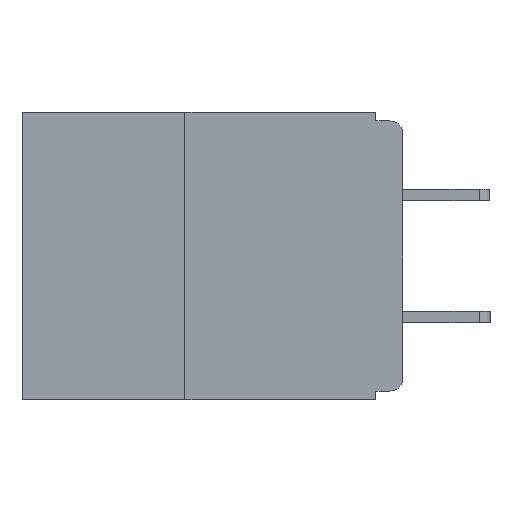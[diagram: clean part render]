
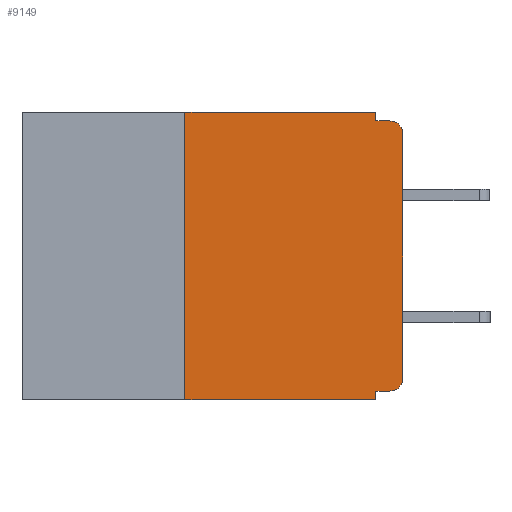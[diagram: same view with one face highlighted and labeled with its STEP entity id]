
A CAD part, left-side view. The second image highlights one B-rep face of the part: STEP entity #9149.
In plain terms, the highlighted planar face has unit normal (-1, 0, 0).
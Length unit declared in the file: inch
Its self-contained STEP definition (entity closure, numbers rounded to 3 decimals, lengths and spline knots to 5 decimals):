
#186 = CARTESIAN_POINT ( 'NONE',  ( 0., 0.25, -0.33 ) ) ;
#391 = DIRECTION ( 'NONE',  ( 0., -1., 0. ) ) ;
#554 = VECTOR ( 'NONE', #391, 39.37008 ) ;
#640 = DIRECTION ( 'NONE',  ( 0., 0., -1. ) ) ;
#1594 = ORIENTED_EDGE ( 'NONE', *, *, #13104, .F. ) ;
#1728 = DIRECTION ( 'NONE',  ( -1., 0., 0. ) ) ;
#1884 = DIRECTION ( 'NONE',  ( 0., 0., -1. ) ) ;
#1994 = CARTESIAN_POINT ( 'NONE',  ( 0., 0.031, -0.33 ) ) ;
#2192 = EDGE_CURVE ( 'NONE', #4188, #13887, #20317, .T. ) ;
#3362 = FACE_OUTER_BOUND ( 'NONE', #13336, .T. ) ;
#3579 = CARTESIAN_POINT ( 'NONE',  ( 0., 0., 0. ) ) ;
#3636 = VERTEX_POINT ( 'NONE', #9568 ) ;
#4188 = VERTEX_POINT ( 'NONE', #186 ) ;
#4613 = CARTESIAN_POINT ( 'NONE',  ( 0., 0.031, -0.01 ) ) ;
#4801 = CARTESIAN_POINT ( 'NONE',  ( 0., 0.015, -0.01 ) ) ;
#4860 = VECTOR ( 'NONE', #6472, 39.37008 ) ;
#4963 = EDGE_CURVE ( 'NONE', #12158, #17159, #18453, .T. ) ;
#5344 = EDGE_CURVE ( 'NONE', #3636, #17159, #9662, .T. ) ;
#6129 = VERTEX_POINT ( 'NONE', #19874 ) ;
#6215 = ORIENTED_EDGE ( 'NONE', *, *, #6844, .T. ) ;
#6323 = VECTOR ( 'NONE', #7617, 39.37008 ) ;
#6472 = DIRECTION ( 'NONE',  ( 0., 1., 0. ) ) ;
#6796 = ORIENTED_EDGE ( 'NONE', *, *, #16630, .F. ) ;
#6844 = EDGE_CURVE ( 'NONE', #16861, #6129, #16753, .T. ) ;
#7011 = VECTOR ( 'NONE', #11040, 39.37008 ) ;
#7360 = CARTESIAN_POINT ( 'NONE',  ( 0., 0.437, 0. ) ) ;
#7577 = LINE ( 'NONE', #1994, #7011 ) ;
#7617 = DIRECTION ( 'NONE',  ( 0., -1., 0. ) ) ;
#7677 = DIRECTION ( 'NONE',  ( -1., 0., 0. ) ) ;
#7740 = VECTOR ( 'NONE', #640, 39.37008 ) ;
#7814 = VECTOR ( 'NONE', #16091, 39.37008 ) ;
#8585 = VECTOR ( 'NONE', #15892, 39.37008 ) ;
#8805 = ORIENTED_EDGE ( 'NONE', *, *, #2192, .T. ) ;
#8962 = VERTEX_POINT ( 'NONE', #12191 ) ;
#9127 = LINE ( 'NONE', #22198, #4860 ) ;
#9149 = ADVANCED_FACE ( 'NONE', ( #3362 ), #12649, .F. ) ;
#9497 = CARTESIAN_POINT ( 'NONE',  ( 0., 0., -0.01 ) ) ;
#9568 = CARTESIAN_POINT ( 'NONE',  ( 0., 0., -0.025 ) ) ;
#9662 = CIRCLE ( 'NONE', #10514, 0.015 ) ;
#9877 = ORIENTED_EDGE ( 'NONE', *, *, #17089, .F. ) ;
#10076 = CARTESIAN_POINT ( 'NONE',  ( 0., 0.031, -0.33 ) ) ;
#10457 = CARTESIAN_POINT ( 'NONE',  ( 0., 0.031, -0.32 ) ) ;
#10514 = AXIS2_PLACEMENT_3D ( 'NONE', #12558, #1728, #14339 ) ;
#10591 = CARTESIAN_POINT ( 'NONE',  ( 0., 0.25, -0.33 ) ) ;
#11040 = DIRECTION ( 'NONE',  ( 0., 0., -1. ) ) ;
#11183 = ORIENTED_EDGE ( 'NONE', *, *, #5344, .T. ) ;
#11469 = ORIENTED_EDGE ( 'NONE', *, *, #4963, .F. ) ;
#12158 = VERTEX_POINT ( 'NONE', #4613 ) ;
#12191 = CARTESIAN_POINT ( 'NONE',  ( 0., 0.031, 0. ) ) ;
#12463 = LINE ( 'NONE', #21855, #7740 ) ;
#12534 = LINE ( 'NONE', #3579, #7814 ) ;
#12558 = CARTESIAN_POINT ( 'NONE',  ( 0., 0.015, -0.025 ) ) ;
#12649 = PLANE ( 'NONE',  #13075 ) ;
#12729 = DIRECTION ( 'NONE',  ( 1., 0., 0. ) ) ;
#13075 = AXIS2_PLACEMENT_3D ( 'NONE', #7360, #12729, #1884 ) ;
#13104 = EDGE_CURVE ( 'NONE', #8962, #12158, #12463, .T. ) ;
#13294 = LINE ( 'NONE', #10591, #8585 ) ;
#13336 = EDGE_LOOP ( 'NONE', ( #20940, #11183, #11469, #1594, #15109, #6796, #8805, #17353, #9877, #6215 ) ) ;
#13887 = VERTEX_POINT ( 'NONE', #10076 ) ;
#14339 = DIRECTION ( 'NONE',  ( 0., 0., -1. ) ) ;
#15109 = ORIENTED_EDGE ( 'NONE', *, *, #16324, .F. ) ;
#15395 = AXIS2_PLACEMENT_3D ( 'NONE', #18224, #7677, #19998 ) ;
#15698 = VECTOR ( 'NONE', #16008, 39.37008 ) ;
#15892 = DIRECTION ( 'NONE',  ( 0., 0., 1. ) ) ;
#16008 = DIRECTION ( 'NONE',  ( 0., -1., 0. ) ) ;
#16091 = DIRECTION ( 'NONE',  ( 0., 0., 1. ) ) ;
#16324 = EDGE_CURVE ( 'NONE', #20480, #8962, #19859, .T. ) ;
#16494 = CARTESIAN_POINT ( 'NONE',  ( 0., 0.015, -0.32 ) ) ;
#16630 = EDGE_CURVE ( 'NONE', #4188, #20480, #13294, .T. ) ;
#16753 = CIRCLE ( 'NONE', #15395, 0.015 ) ;
#16861 = VERTEX_POINT ( 'NONE', #16494 ) ;
#17089 = EDGE_CURVE ( 'NONE', #16861, #20048, #9127, .T. ) ;
#17159 = VERTEX_POINT ( 'NONE', #4801 ) ;
#17204 = CARTESIAN_POINT ( 'NONE',  ( 0., 0.25, 0. ) ) ;
#17353 = ORIENTED_EDGE ( 'NONE', *, *, #21695, .F. ) ;
#18156 = CARTESIAN_POINT ( 'NONE',  ( 0., 0.437, 0. ) ) ;
#18224 = CARTESIAN_POINT ( 'NONE',  ( 0., 0.015, -0.305 ) ) ;
#18453 = LINE ( 'NONE', #9497, #554 ) ;
#19859 = LINE ( 'NONE', #18156, #6323 ) ;
#19874 = CARTESIAN_POINT ( 'NONE',  ( 0., 0., -0.305 ) ) ;
#19998 = DIRECTION ( 'NONE',  ( 0., 0., -1. ) ) ;
#20048 = VERTEX_POINT ( 'NONE', #10457 ) ;
#20317 = LINE ( 'NONE', #22821, #15698 ) ;
#20480 = VERTEX_POINT ( 'NONE', #17204 ) ;
#20940 = ORIENTED_EDGE ( 'NONE', *, *, #21288, .T. ) ;
#21288 = EDGE_CURVE ( 'NONE', #6129, #3636, #12534, .T. ) ;
#21695 = EDGE_CURVE ( 'NONE', #20048, #13887, #7577, .T. ) ;
#21855 = CARTESIAN_POINT ( 'NONE',  ( 0., 0.031, 0. ) ) ;
#22198 = CARTESIAN_POINT ( 'NONE',  ( 0., 0., -0.32 ) ) ;
#22821 = CARTESIAN_POINT ( 'NONE',  ( 0., 0.437, -0.33 ) ) ;
